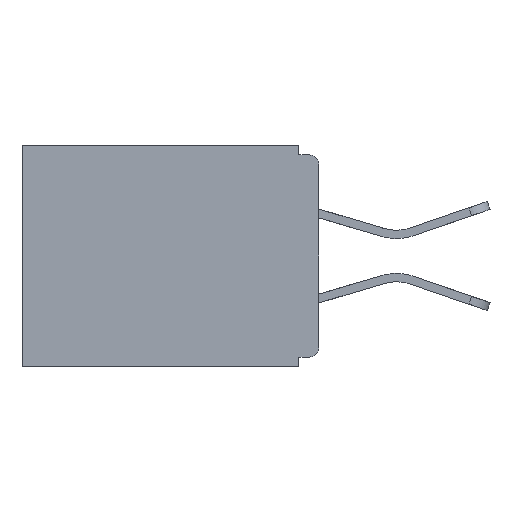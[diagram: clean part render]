
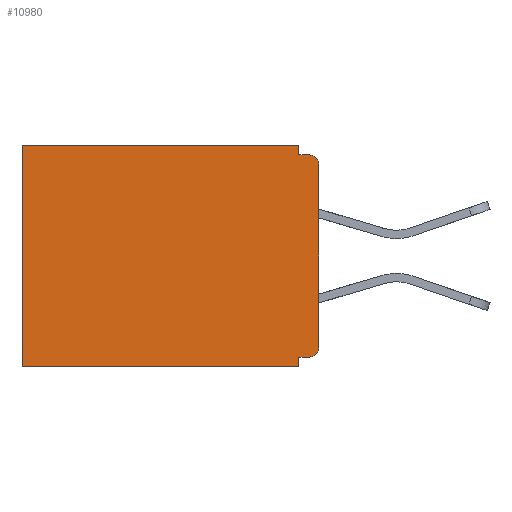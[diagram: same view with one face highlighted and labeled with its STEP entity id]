
A CAD part, left-side view. The second image highlights one B-rep face of the part: STEP entity #10980.
In plain terms, the highlighted planar face has unit normal (-1, 0, 0).
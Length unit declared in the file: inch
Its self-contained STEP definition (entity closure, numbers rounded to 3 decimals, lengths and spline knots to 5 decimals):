
#250 = EDGE_CURVE ( 'NONE', #6580, #6140, #17755, .T. ) ;
#443 = DIRECTION ( 'NONE',  ( 0., 1., 0. ) ) ;
#1023 = EDGE_CURVE ( 'NONE', #5024, #1098, #16640, .T. ) ;
#1098 = VERTEX_POINT ( 'NONE', #13083 ) ;
#2091 = DIRECTION ( 'NONE',  ( 0., -1., 0. ) ) ;
#2734 = CARTESIAN_POINT ( 'NONE',  ( 0.298, 0.015, -0.015 ) ) ;
#2798 = LINE ( 'NONE', #5736, #6055 ) ;
#3080 = CIRCLE ( 'NONE', #3302, 0.015 ) ;
#3116 = CARTESIAN_POINT ( 'NONE',  ( 0.298, 0.015, -0.328 ) ) ;
#3135 = CARTESIAN_POINT ( 'NONE',  ( 0.298, 0., -0.03 ) ) ;
#3188 = CARTESIAN_POINT ( 'NONE',  ( 0.298, 0., -0.343 ) ) ;
#3302 = AXIS2_PLACEMENT_3D ( 'NONE', #6443, #12185, #16153 ) ;
#3535 = LINE ( 'NONE', #7094, #5455 ) ;
#3546 = DIRECTION ( 'NONE',  ( 1., 0., 0. ) ) ;
#3581 = CARTESIAN_POINT ( 'NONE',  ( 0.298, 0.46, 0. ) ) ;
#3965 = CARTESIAN_POINT ( 'NONE',  ( 0.298, 0.031, -0.343 ) ) ;
#4074 = DIRECTION ( 'NONE',  ( -1., 0., 0. ) ) ;
#4372 = DIRECTION ( 'NONE',  ( 0., 1., 0. ) ) ;
#4421 = VECTOR ( 'NONE', #10426, 39.37008 ) ;
#4502 = ORIENTED_EDGE ( 'NONE', *, *, #14383, .F. ) ;
#4811 = PLANE ( 'NONE',  #10314 ) ;
#5024 = VERTEX_POINT ( 'NONE', #3116 ) ;
#5120 = DIRECTION ( 'NONE',  ( 0., 0., -1. ) ) ;
#5455 = VECTOR ( 'NONE', #12651, 39.37008 ) ;
#5533 = CARTESIAN_POINT ( 'NONE',  ( 0.298, 0., -0.015 ) ) ;
#5724 = ORIENTED_EDGE ( 'NONE', *, *, #16878, .F. ) ;
#5736 = CARTESIAN_POINT ( 'NONE',  ( 0.298, 0., 0. ) ) ;
#5815 = LINE ( 'NONE', #15351, #17512 ) ;
#5875 = ORIENTED_EDGE ( 'NONE', *, *, #11830, .T. ) ;
#5973 = ORIENTED_EDGE ( 'NONE', *, *, #6677, .T. ) ;
#5991 = ORIENTED_EDGE ( 'NONE', *, *, #7417, .F. ) ;
#6055 = VECTOR ( 'NONE', #8562, 39.37008 ) ;
#6140 = VERTEX_POINT ( 'NONE', #2734 ) ;
#6397 = VERTEX_POINT ( 'NONE', #14547 ) ;
#6443 = CARTESIAN_POINT ( 'NONE',  ( 0.298, 0.015, -0.03 ) ) ;
#6465 = VERTEX_POINT ( 'NONE', #17577 ) ;
#6580 = VERTEX_POINT ( 'NONE', #8726 ) ;
#6640 = VECTOR ( 'NONE', #443, 39.37008 ) ;
#6677 = EDGE_CURVE ( 'NONE', #15855, #6140, #3080, .T. ) ;
#7094 = CARTESIAN_POINT ( 'NONE',  ( 0.298, 0.031, -0.343 ) ) ;
#7150 = LINE ( 'NONE', #11233, #17540 ) ;
#7233 = FACE_OUTER_BOUND ( 'NONE', #17414, .T. ) ;
#7417 = EDGE_CURVE ( 'NONE', #12807, #17395, #3535, .T. ) ;
#7483 = VERTEX_POINT ( 'NONE', #14823 ) ;
#7497 = DIRECTION ( 'NONE',  ( 0., 0., -1. ) ) ;
#8279 = EDGE_CURVE ( 'NONE', #5024, #12807, #7150, .T. ) ;
#8407 = AXIS2_PLACEMENT_3D ( 'NONE', #11176, #4074, #11237 ) ;
#8460 = EDGE_CURVE ( 'NONE', #6465, #7483, #2798, .T. ) ;
#8562 = DIRECTION ( 'NONE',  ( 0., 1., 0. ) ) ;
#8726 = CARTESIAN_POINT ( 'NONE',  ( 0.298, 0.031, -0.015 ) ) ;
#10166 = LINE ( 'NONE', #3188, #6640 ) ;
#10314 = AXIS2_PLACEMENT_3D ( 'NONE', #15918, #3546, #7497 ) ;
#10426 = DIRECTION ( 'NONE',  ( 0., 0., -1. ) ) ;
#10980 = ADVANCED_FACE ( 'NONE', ( #7233 ), #4811, .F. ) ;
#11176 = CARTESIAN_POINT ( 'NONE',  ( 0.298, 0.015, -0.313 ) ) ;
#11233 = CARTESIAN_POINT ( 'NONE',  ( 0.298, 0., -0.328 ) ) ;
#11237 = DIRECTION ( 'NONE',  ( 0., 0., -1. ) ) ;
#11312 = DIRECTION ( 'NONE',  ( 0., 0., -1. ) ) ;
#11459 = ORIENTED_EDGE ( 'NONE', *, *, #1023, .T. ) ;
#11830 = EDGE_CURVE ( 'NONE', #7483, #6397, #17173, .T. ) ;
#12087 = CARTESIAN_POINT ( 'NONE',  ( 0.298, 0.031, -0.343 ) ) ;
#12185 = DIRECTION ( 'NONE',  ( -1., 0., 0. ) ) ;
#12252 = ORIENTED_EDGE ( 'NONE', *, *, #250, .F. ) ;
#12651 = DIRECTION ( 'NONE',  ( 0., 0., -1. ) ) ;
#12807 = VERTEX_POINT ( 'NONE', #14337 ) ;
#13083 = CARTESIAN_POINT ( 'NONE',  ( 0.298, 0., -0.313 ) ) ;
#13089 = LINE ( 'NONE', #12087, #16097 ) ;
#13165 = ORIENTED_EDGE ( 'NONE', *, *, #8460, .T. ) ;
#13211 = VECTOR ( 'NONE', #2091, 39.37008 ) ;
#14337 = CARTESIAN_POINT ( 'NONE',  ( 0.298, 0.031, -0.328 ) ) ;
#14383 = EDGE_CURVE ( 'NONE', #15855, #1098, #5815, .T. ) ;
#14413 = ORIENTED_EDGE ( 'NONE', *, *, #8279, .F. ) ;
#14547 = CARTESIAN_POINT ( 'NONE',  ( 0.298, 0.46, -0.343 ) ) ;
#14796 = EDGE_CURVE ( 'NONE', #17395, #6397, #10166, .T. ) ;
#14823 = CARTESIAN_POINT ( 'NONE',  ( 0.298, 0.46, 0. ) ) ;
#15351 = CARTESIAN_POINT ( 'NONE',  ( 0.298, 0., 0. ) ) ;
#15855 = VERTEX_POINT ( 'NONE', #3135 ) ;
#15866 = ORIENTED_EDGE ( 'NONE', *, *, #14796, .F. ) ;
#15918 = CARTESIAN_POINT ( 'NONE',  ( 0.298, 0., 0. ) ) ;
#16097 = VECTOR ( 'NONE', #5120, 39.37008 ) ;
#16153 = DIRECTION ( 'NONE',  ( 0., 0., -1. ) ) ;
#16640 = CIRCLE ( 'NONE', #8407, 0.015 ) ;
#16878 = EDGE_CURVE ( 'NONE', #6465, #6580, #13089, .T. ) ;
#17173 = LINE ( 'NONE', #3581, #4421 ) ;
#17395 = VERTEX_POINT ( 'NONE', #3965 ) ;
#17414 = EDGE_LOOP ( 'NONE', ( #5973, #12252, #5724, #13165, #5875, #15866, #5991, #14413, #11459, #4502 ) ) ;
#17512 = VECTOR ( 'NONE', #11312, 39.37008 ) ;
#17540 = VECTOR ( 'NONE', #4372, 39.37008 ) ;
#17577 = CARTESIAN_POINT ( 'NONE',  ( 0.298, 0.031, 0. ) ) ;
#17755 = LINE ( 'NONE', #5533, #13211 ) ;
